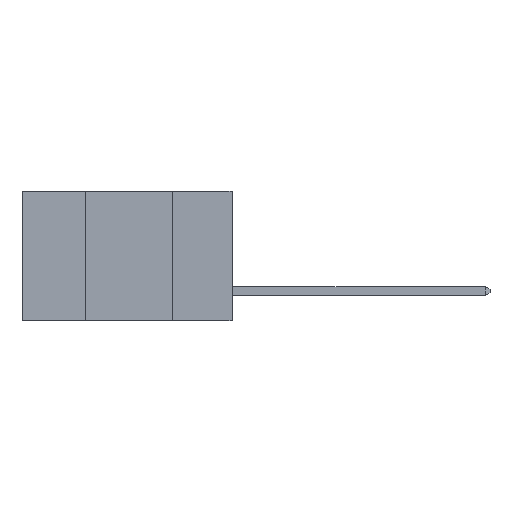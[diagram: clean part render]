
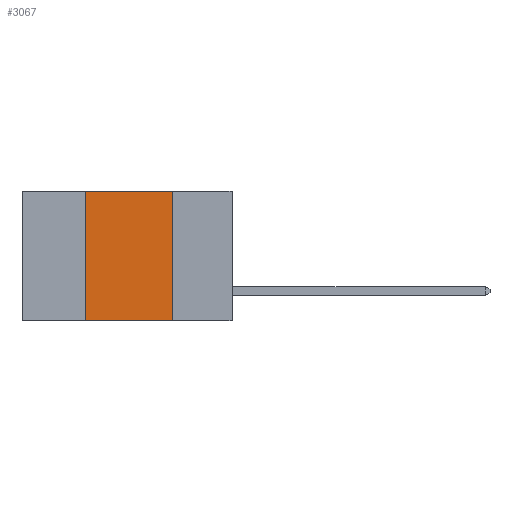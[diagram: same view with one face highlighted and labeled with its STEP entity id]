
A CAD part, left-side view. The second image highlights one B-rep face of the part: STEP entity #3067.
In plain terms, the highlighted planar face has unit normal (-1, 0, 0).
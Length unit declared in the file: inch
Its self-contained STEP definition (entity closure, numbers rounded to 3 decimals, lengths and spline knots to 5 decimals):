
#739 = DIRECTION ( 'NONE',  ( 0., 0., -1. ) ) ;
#1087 = ORIENTED_EDGE ( 'NONE', *, *, #8824, .T. ) ;
#1126 = VECTOR ( 'NONE', #12644, 39.37008 ) ;
#1145 = ORIENTED_EDGE ( 'NONE', *, *, #4333, .F. ) ;
#1205 = VERTEX_POINT ( 'NONE', #5134 ) ;
#1263 = AXIS2_PLACEMENT_3D ( 'NONE', #8615, #1617, #739 ) ;
#1617 = DIRECTION ( 'NONE',  ( 1., 0., 0. ) ) ;
#2709 = DIRECTION ( 'NONE',  ( 0., 0., 1. ) ) ;
#2724 = CARTESIAN_POINT ( 'NONE',  ( 0., 0.42, 0. ) ) ;
#3067 = ADVANCED_FACE ( 'NONE', ( #8899 ), #8296, .F. ) ;
#3178 = VERTEX_POINT ( 'NONE', #7051 ) ;
#4141 = LINE ( 'NONE', #4964, #1126 ) ;
#4249 = ORIENTED_EDGE ( 'NONE', *, *, #9871, .F. ) ;
#4279 = ORIENTED_EDGE ( 'NONE', *, *, #5097, .F. ) ;
#4333 = EDGE_CURVE ( 'NONE', #3178, #1205, #8961, .T. ) ;
#4462 = DIRECTION ( 'NONE',  ( 0., -1., 0. ) ) ;
#4964 = CARTESIAN_POINT ( 'NONE',  ( 0., 0.17, 0. ) ) ;
#5097 = EDGE_CURVE ( 'NONE', #10254, #3178, #6469, .T. ) ;
#5134 = CARTESIAN_POINT ( 'NONE',  ( 0., 0.17, 0. ) ) ;
#5466 = VECTOR ( 'NONE', #6487, 39.37008 ) ;
#5669 = CARTESIAN_POINT ( 'NONE',  ( 0., 0.6, 0. ) ) ;
#5758 = LINE ( 'NONE', #12161, #5466 ) ;
#6469 = LINE ( 'NONE', #2724, #11524 ) ;
#6487 = DIRECTION ( 'NONE',  ( 0., -1., 0. ) ) ;
#6876 = VERTEX_POINT ( 'NONE', #8191 ) ;
#7051 = CARTESIAN_POINT ( 'NONE',  ( 0., 0.42, 0. ) ) ;
#8191 = CARTESIAN_POINT ( 'NONE',  ( 0., 0.17, -0.37 ) ) ;
#8296 = PLANE ( 'NONE',  #1263 ) ;
#8583 = CARTESIAN_POINT ( 'NONE',  ( 0., 0.42, -0.37 ) ) ;
#8615 = CARTESIAN_POINT ( 'NONE',  ( 0., 0.6, 0. ) ) ;
#8824 = EDGE_CURVE ( 'NONE', #10254, #6876, #5758, .T. ) ;
#8899 = FACE_OUTER_BOUND ( 'NONE', #10727, .T. ) ;
#8961 = LINE ( 'NONE', #5669, #11386 ) ;
#9871 = EDGE_CURVE ( 'NONE', #1205, #6876, #4141, .T. ) ;
#10254 = VERTEX_POINT ( 'NONE', #8583 ) ;
#10727 = EDGE_LOOP ( 'NONE', ( #4249, #1145, #4279, #1087 ) ) ;
#11386 = VECTOR ( 'NONE', #4462, 39.37008 ) ;
#11524 = VECTOR ( 'NONE', #2709, 39.37008 ) ;
#12161 = CARTESIAN_POINT ( 'NONE',  ( 0., 0.6, -0.37 ) ) ;
#12644 = DIRECTION ( 'NONE',  ( 0., 0., -1. ) ) ;
